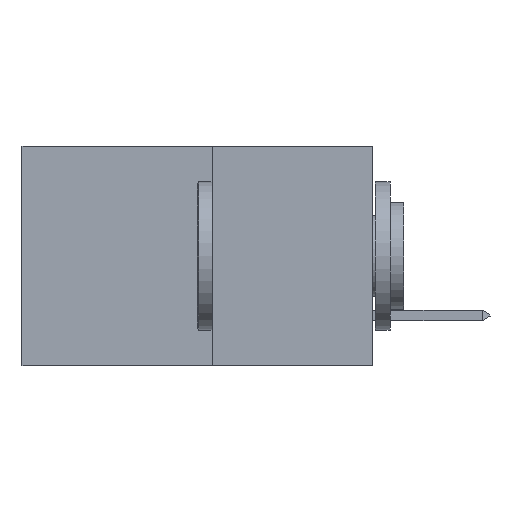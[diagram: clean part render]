
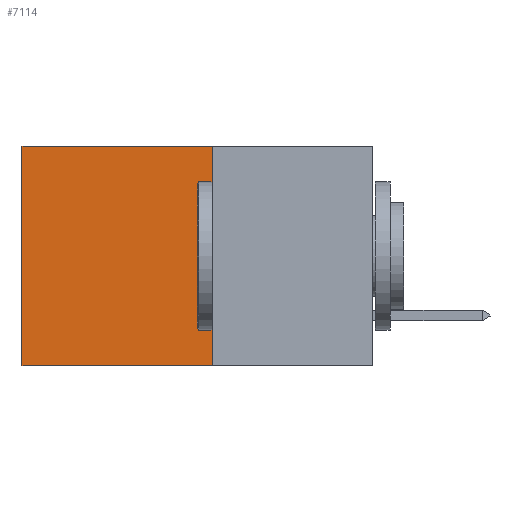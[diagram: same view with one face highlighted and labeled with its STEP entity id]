
A CAD part, left-side view. The second image highlights one B-rep face of the part: STEP entity #7114.
In plain terms, the highlighted planar face has unit normal (-1, 0, 0).
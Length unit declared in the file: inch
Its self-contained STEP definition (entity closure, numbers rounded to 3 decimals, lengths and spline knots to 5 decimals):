
#546 = ORIENTED_EDGE ( 'NONE', *, *, #18227, .F. ) ;
#572 = LINE ( 'NONE', #9323, #12427 ) ;
#702 = VECTOR ( 'NONE', #3985, 39.37008 ) ;
#1805 = CARTESIAN_POINT ( 'NONE',  ( 0.277, 0.59, 0. ) ) ;
#1880 = CARTESIAN_POINT ( 'NONE',  ( 0.277, 0.59, -0.37 ) ) ;
#2172 = VERTEX_POINT ( 'NONE', #1880 ) ;
#2696 = VECTOR ( 'NONE', #11478, 39.37008 ) ;
#2888 = EDGE_CURVE ( 'NONE', #12232, #13171, #572, .T. ) ;
#2954 = VECTOR ( 'NONE', #9465, 39.37008 ) ;
#3985 = DIRECTION ( 'NONE',  ( 0., 0., -1. ) ) ;
#4186 = CARTESIAN_POINT ( 'NONE',  ( 0.277, 0.59, -0.37 ) ) ;
#5974 = EDGE_CURVE ( 'NONE', #8777, #2172, #7684, .T. ) ;
#7114 = ADVANCED_FACE ( 'NONE', ( #13899 ), #17369, .F. ) ;
#7488 = CARTESIAN_POINT ( 'NONE',  ( 0.277, 0.27, -0.37 ) ) ;
#7684 = LINE ( 'NONE', #4186, #702 ) ;
#7756 = EDGE_CURVE ( 'NONE', #12232, #8777, #14114, .T. ) ;
#7978 = CARTESIAN_POINT ( 'NONE',  ( 0.277, 0.27, -0.37 ) ) ;
#8777 = VERTEX_POINT ( 'NONE', #1805 ) ;
#9267 = ORIENTED_EDGE ( 'NONE', *, *, #5974, .T. ) ;
#9323 = CARTESIAN_POINT ( 'NONE',  ( 0.277, 0.27, -0.37 ) ) ;
#9465 = DIRECTION ( 'NONE',  ( 0., 1., 0. ) ) ;
#9793 = CARTESIAN_POINT ( 'NONE',  ( 0.277, 0.27, 0. ) ) ;
#10893 = LINE ( 'NONE', #7978, #2954 ) ;
#11478 = DIRECTION ( 'NONE',  ( 0., 1., 0. ) ) ;
#11534 = CARTESIAN_POINT ( 'NONE',  ( 0.277, 0.27, 0. ) ) ;
#11555 = EDGE_LOOP ( 'NONE', ( #9267, #546, #17480, #17551 ) ) ;
#12232 = VERTEX_POINT ( 'NONE', #9793 ) ;
#12427 = VECTOR ( 'NONE', #16860, 39.37008 ) ;
#13171 = VERTEX_POINT ( 'NONE', #7488 ) ;
#13899 = FACE_OUTER_BOUND ( 'NONE', #11555, .T. ) ;
#14114 = LINE ( 'NONE', #11534, #2696 ) ;
#16238 = AXIS2_PLACEMENT_3D ( 'NONE', #17109, #17106, #17086 ) ;
#16860 = DIRECTION ( 'NONE',  ( 0., 0., -1. ) ) ;
#17086 = DIRECTION ( 'NONE',  ( 0., 0., -1. ) ) ;
#17106 = DIRECTION ( 'NONE',  ( 1., 0., 0. ) ) ;
#17109 = CARTESIAN_POINT ( 'NONE',  ( 0.277, 0.27, -0.37 ) ) ;
#17369 = PLANE ( 'NONE',  #16238 ) ;
#17480 = ORIENTED_EDGE ( 'NONE', *, *, #2888, .F. ) ;
#17551 = ORIENTED_EDGE ( 'NONE', *, *, #7756, .T. ) ;
#18227 = EDGE_CURVE ( 'NONE', #13171, #2172, #10893, .T. ) ;
